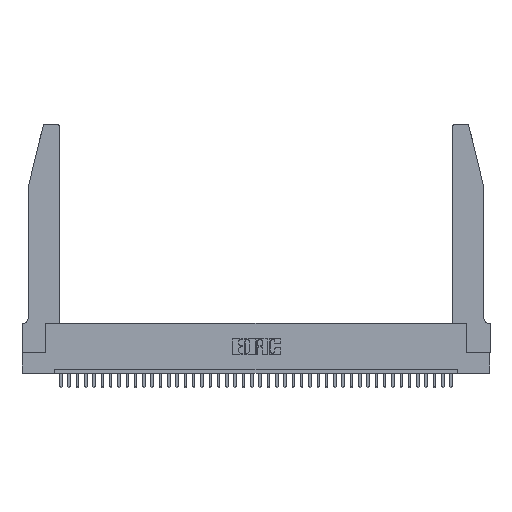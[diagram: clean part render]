
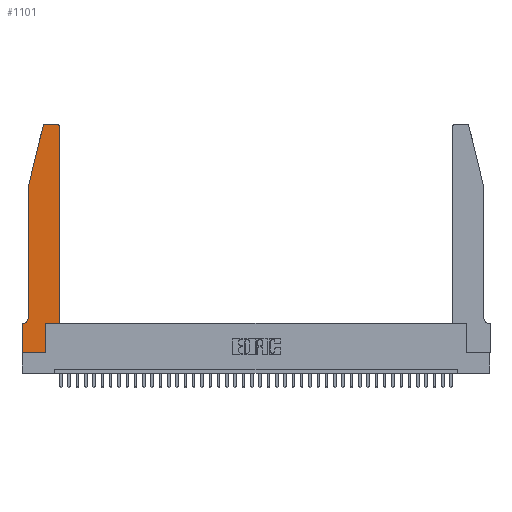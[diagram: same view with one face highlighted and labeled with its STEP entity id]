
A CAD part, top view. The second image highlights one B-rep face of the part: STEP entity #1101.
In plain terms, the highlighted planar face has unit normal (0, 0, 1).
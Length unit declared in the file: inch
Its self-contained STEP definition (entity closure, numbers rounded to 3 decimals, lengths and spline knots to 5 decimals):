
#44 = DIRECTION ( 'NONE',  ( 1., 0., 0. ) ) ;
#236 = LINE ( 'NONE', #10863, #30444 ) ;
#801 = LINE ( 'NONE', #30410, #24629 ) ;
#1101 = ADVANCED_FACE ( 'NONE', ( #37439 ), #16820, .T. ) ;
#1343 = DIRECTION ( 'NONE',  ( 0., 1., 0. ) ) ;
#2377 = CARTESIAN_POINT ( 'NONE',  ( 0.25487, 2.72718, 0.37 ) ) ;
#2467 = VECTOR ( 'NONE', #9688, 39.37008 ) ;
#2529 = DIRECTION ( 'NONE',  ( -1., 0., 0. ) ) ;
#2669 = CARTESIAN_POINT ( 'NONE',  ( 0.4505, 0.35, 0.37 ) ) ;
#3031 = LINE ( 'NONE', #2669, #29300 ) ;
#4043 = DIRECTION ( 'NONE',  ( 0., 0., 1. ) ) ;
#5409 = VERTEX_POINT ( 'NONE', #2377 ) ;
#5842 = CARTESIAN_POINT ( 'NONE',  ( 0.4205, 2.72, 0.37 ) ) ;
#7730 = ORIENTED_EDGE ( 'NONE', *, *, #34598, .T. ) ;
#8474 = ORIENTED_EDGE ( 'NONE', *, *, #25415, .T. ) ;
#8753 = CARTESIAN_POINT ( 'NONE',  ( 0.4505, 0.35, 0.37 ) ) ;
#9688 = DIRECTION ( 'NONE',  ( -1., 0., 0. ) ) ;
#10130 = EDGE_CURVE ( 'NONE', #30762, #20930, #27036, .T. ) ;
#10151 = CARTESIAN_POINT ( 'NONE',  ( 0.284, 2.72, 0.37 ) ) ;
#10707 = LINE ( 'NONE', #22352, #2467 ) ;
#10722 = VECTOR ( 'NONE', #1343, 39.37008 ) ;
#10863 = CARTESIAN_POINT ( 'NONE',  ( 0.0755, 2., 0.37 ) ) ;
#11720 = CARTESIAN_POINT ( 'NONE',  ( 0.0055, 0.42, 0.37 ) ) ;
#12267 = EDGE_CURVE ( 'NONE', #18439, #15330, #3031, .T. ) ;
#13285 = DIRECTION ( 'NONE',  ( 1., 0., 0. ) ) ;
#13413 = CARTESIAN_POINT ( 'NONE',  ( 0., 0.35, 0.37 ) ) ;
#13423 = AXIS2_PLACEMENT_3D ( 'NONE', #35161, #4043, #29052 ) ;
#13484 = VERTEX_POINT ( 'NONE', #20719 ) ;
#14058 = DIRECTION ( 'NONE',  ( -0.239, -0.971, 0. ) ) ;
#14396 = DIRECTION ( 'NONE',  ( 0., -1., 0. ) ) ;
#14783 = ORIENTED_EDGE ( 'NONE', *, *, #36824, .T. ) ;
#14870 = DIRECTION ( 'NONE',  ( 1., 0., 0. ) ) ;
#14881 = VECTOR ( 'NONE', #31145, 39.37008 ) ;
#15309 = EDGE_LOOP ( 'NONE', ( #15730, #20905, #27415, #8474, #36753, #22192, #15975, #20876, #14783, #28456, #38778, #7730 ) ) ;
#15330 = VERTEX_POINT ( 'NONE', #8753 ) ;
#15730 = ORIENTED_EDGE ( 'NONE', *, *, #20806, .T. ) ;
#15975 = ORIENTED_EDGE ( 'NONE', *, *, #10130, .T. ) ;
#16359 = CARTESIAN_POINT ( 'NONE',  ( 0., 0., 0.37 ) ) ;
#16820 = PLANE ( 'NONE',  #13423 ) ;
#16997 = VECTOR ( 'NONE', #33832, 39.37008 ) ;
#17308 = VERTEX_POINT ( 'NONE', #23107 ) ;
#18439 = VERTEX_POINT ( 'NONE', #19185 ) ;
#19116 = AXIS2_PLACEMENT_3D ( 'NONE', #10151, #22537, #13285 ) ;
#19185 = CARTESIAN_POINT ( 'NONE',  ( 0.2865, 0.35, 0.37 ) ) ;
#19943 = CARTESIAN_POINT ( 'NONE',  ( 0.4505, 0.35, 0.37 ) ) ;
#20358 = EDGE_CURVE ( 'NONE', #15330, #21246, #37457, .T. ) ;
#20435 = LINE ( 'NONE', #16359, #27689 ) ;
#20686 = EDGE_CURVE ( 'NONE', #37174, #30762, #10707, .T. ) ;
#20719 = CARTESIAN_POINT ( 'NONE',  ( 0.284, 2.75, 0.37 ) ) ;
#20806 = EDGE_CURVE ( 'NONE', #37817, #13484, #25207, .T. ) ;
#20876 = ORIENTED_EDGE ( 'NONE', *, *, #32876, .T. ) ;
#20905 = ORIENTED_EDGE ( 'NONE', *, *, #33497, .T. ) ;
#20930 = VERTEX_POINT ( 'NONE', #39243 ) ;
#21246 = VERTEX_POINT ( 'NONE', #22344 ) ;
#22192 = ORIENTED_EDGE ( 'NONE', *, *, #20686, .T. ) ;
#22344 = CARTESIAN_POINT ( 'NONE',  ( 0.4505, 2.72, 0.37 ) ) ;
#22352 = CARTESIAN_POINT ( 'NONE',  ( 0.0755, 0.35, 0.37 ) ) ;
#22537 = DIRECTION ( 'NONE',  ( 0., 0., 1. ) ) ;
#23029 = DIRECTION ( 'NONE',  ( 1., 0., 0. ) ) ;
#23107 = CARTESIAN_POINT ( 'NONE',  ( 0.0755, 0.42, 0.37 ) ) ;
#24455 = EDGE_CURVE ( 'NONE', #17308, #37174, #34852, .T. ) ;
#24629 = VECTOR ( 'NONE', #14058, 39.37008 ) ;
#25101 = AXIS2_PLACEMENT_3D ( 'NONE', #5842, #37261, #44 ) ;
#25207 = LINE ( 'NONE', #35290, #33092 ) ;
#25411 = VERTEX_POINT ( 'NONE', #39269 ) ;
#25415 = EDGE_CURVE ( 'NONE', #25411, #17308, #236, .T. ) ;
#27036 = LINE ( 'NONE', #39595, #14881 ) ;
#27368 = DIRECTION ( 'NONE',  ( 0., 0., -1. ) ) ;
#27415 = ORIENTED_EDGE ( 'NONE', *, *, #38138, .T. ) ;
#27689 = VECTOR ( 'NONE', #23029, 39.37008 ) ;
#28456 = ORIENTED_EDGE ( 'NONE', *, *, #12267, .T. ) ;
#29052 = DIRECTION ( 'NONE',  ( 1., 0., 0. ) ) ;
#29300 = VECTOR ( 'NONE', #14870, 39.37008 ) ;
#30410 = CARTESIAN_POINT ( 'NONE',  ( 0.0755, 2., 0.37 ) ) ;
#30444 = VECTOR ( 'NONE', #14396, 39.37008 ) ;
#30704 = CARTESIAN_POINT ( 'NONE',  ( 0.4205, 2.75, 0.37 ) ) ;
#30762 = VERTEX_POINT ( 'NONE', #13413 ) ;
#30767 = CIRCLE ( 'NONE', #25101, 0.03 ) ;
#30924 = CARTESIAN_POINT ( 'NONE',  ( 0.2865, 0., 0.37 ) ) ;
#31145 = DIRECTION ( 'NONE',  ( 0., -1., 0. ) ) ;
#31274 = VERTEX_POINT ( 'NONE', #30924 ) ;
#32329 = CARTESIAN_POINT ( 'NONE',  ( 0.0055, 0.35, 0.37 ) ) ;
#32876 = EDGE_CURVE ( 'NONE', #20930, #31274, #20435, .T. ) ;
#33092 = VECTOR ( 'NONE', #38731, 39.37008 ) ;
#33497 = EDGE_CURVE ( 'NONE', #13484, #5409, #36407, .T. ) ;
#33832 = DIRECTION ( 'NONE',  ( 0., 1., 0. ) ) ;
#34598 = EDGE_CURVE ( 'NONE', #21246, #37817, #30767, .T. ) ;
#34852 = CIRCLE ( 'NONE', #36905, 0.07 ) ;
#35161 = CARTESIAN_POINT ( 'NONE',  ( 0., 0.35, 0.37 ) ) ;
#35290 = CARTESIAN_POINT ( 'NONE',  ( 0.2605, 2.75, 0.37 ) ) ;
#35964 = LINE ( 'NONE', #40043, #16997 ) ;
#36407 = CIRCLE ( 'NONE', #19116, 0.03 ) ;
#36753 = ORIENTED_EDGE ( 'NONE', *, *, #24455, .T. ) ;
#36824 = EDGE_CURVE ( 'NONE', #31274, #18439, #35964, .T. ) ;
#36905 = AXIS2_PLACEMENT_3D ( 'NONE', #11720, #27368, #2529 ) ;
#37174 = VERTEX_POINT ( 'NONE', #32329 ) ;
#37261 = DIRECTION ( 'NONE',  ( 0., 0., 1. ) ) ;
#37439 = FACE_OUTER_BOUND ( 'NONE', #15309, .T. ) ;
#37457 = LINE ( 'NONE', #19943, #10722 ) ;
#37817 = VERTEX_POINT ( 'NONE', #30704 ) ;
#38138 = EDGE_CURVE ( 'NONE', #5409, #25411, #801, .T. ) ;
#38731 = DIRECTION ( 'NONE',  ( -1., 0., 0. ) ) ;
#38778 = ORIENTED_EDGE ( 'NONE', *, *, #20358, .T. ) ;
#39243 = CARTESIAN_POINT ( 'NONE',  ( 0., 0., 0.37 ) ) ;
#39269 = CARTESIAN_POINT ( 'NONE',  ( 0.0755, 2., 0.37 ) ) ;
#39595 = CARTESIAN_POINT ( 'NONE',  ( 0., 0., 0.37 ) ) ;
#40043 = CARTESIAN_POINT ( 'NONE',  ( 0.2865, 0.35, 0.37 ) ) ;
